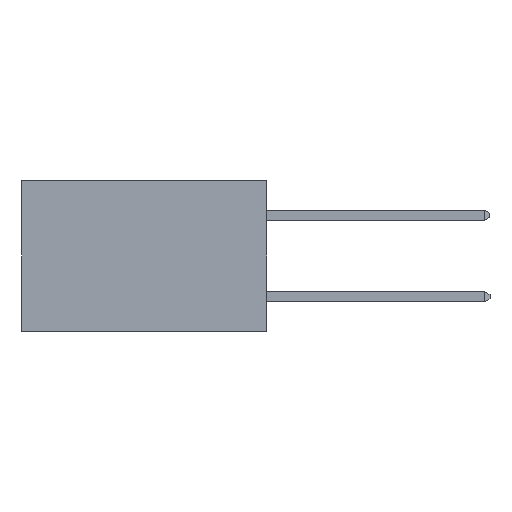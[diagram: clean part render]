
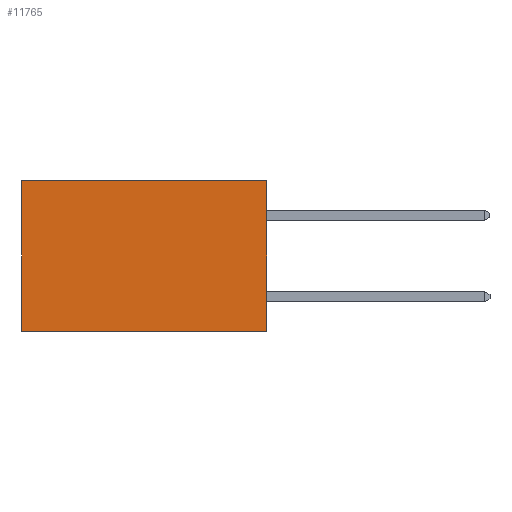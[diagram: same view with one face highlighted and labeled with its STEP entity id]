
A CAD part, left-side view. The second image highlights one B-rep face of the part: STEP entity #11765.
In plain terms, the highlighted planar face has unit normal (-1, 0, 0).
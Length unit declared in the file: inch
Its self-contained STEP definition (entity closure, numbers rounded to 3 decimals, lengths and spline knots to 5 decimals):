
#58 = EDGE_CURVE ( 'NONE', #2391, #2931, #9370, .T. ) ;
#368 = DIRECTION ( 'NONE',  ( 0., 0., -1. ) ) ;
#513 = LINE ( 'NONE', #10757, #8063 ) ;
#1424 = LINE ( 'NONE', #6221, #7368 ) ;
#1634 = EDGE_CURVE ( 'NONE', #2931, #11163, #513, .T. ) ;
#1973 = EDGE_CURVE ( 'NONE', #2391, #8317, #9157, .T. ) ;
#2129 = DIRECTION ( 'NONE',  ( 0., 0., -1. ) ) ;
#2391 = VERTEX_POINT ( 'NONE', #13063 ) ;
#2931 = VERTEX_POINT ( 'NONE', #6387 ) ;
#2952 = CARTESIAN_POINT ( 'NONE',  ( 0.2875, 0., 0. ) ) ;
#3901 = DIRECTION ( 'NONE',  ( 0., 1., 0. ) ) ;
#3923 = VECTOR ( 'NONE', #3943, 39.37008 ) ;
#3943 = DIRECTION ( 'NONE',  ( 0., 0., -1. ) ) ;
#4348 = ORIENTED_EDGE ( 'NONE', *, *, #6949, .T. ) ;
#4667 = DIRECTION ( 'NONE',  ( 1., 0., 0. ) ) ;
#6221 = CARTESIAN_POINT ( 'NONE',  ( 0.2875, 0.6, 0. ) ) ;
#6387 = CARTESIAN_POINT ( 'NONE',  ( 0.2875, 0., -0.37 ) ) ;
#6742 = DIRECTION ( 'NONE',  ( 0., 1., 0. ) ) ;
#6826 = ORIENTED_EDGE ( 'NONE', *, *, #58, .F. ) ;
#6949 = EDGE_CURVE ( 'NONE', #8317, #11163, #1424, .T. ) ;
#7071 = EDGE_LOOP ( 'NONE', ( #4348, #9352, #6826, #9397 ) ) ;
#7368 = VECTOR ( 'NONE', #2129, 39.37008 ) ;
#8063 = VECTOR ( 'NONE', #6742, 39.37008 ) ;
#8317 = VERTEX_POINT ( 'NONE', #9177 ) ;
#9157 = LINE ( 'NONE', #12141, #9624 ) ;
#9177 = CARTESIAN_POINT ( 'NONE',  ( 0.2875, 0.6, 0. ) ) ;
#9352 = ORIENTED_EDGE ( 'NONE', *, *, #1634, .F. ) ;
#9370 = LINE ( 'NONE', #2952, #3923 ) ;
#9397 = ORIENTED_EDGE ( 'NONE', *, *, #1973, .T. ) ;
#9600 = FACE_OUTER_BOUND ( 'NONE', #7071, .T. ) ;
#9624 = VECTOR ( 'NONE', #3901, 39.37008 ) ;
#9629 = AXIS2_PLACEMENT_3D ( 'NONE', #9697, #4667, #368 ) ;
#9697 = CARTESIAN_POINT ( 'NONE',  ( 0.2875, 0., 0. ) ) ;
#10757 = CARTESIAN_POINT ( 'NONE',  ( 0.2875, 0., -0.37 ) ) ;
#10796 = PLANE ( 'NONE',  #9629 ) ;
#11163 = VERTEX_POINT ( 'NONE', #12715 ) ;
#11765 = ADVANCED_FACE ( 'NONE', ( #9600 ), #10796, .F. ) ;
#12141 = CARTESIAN_POINT ( 'NONE',  ( 0.2875, 0., 0. ) ) ;
#12715 = CARTESIAN_POINT ( 'NONE',  ( 0.2875, 0.6, -0.37 ) ) ;
#13063 = CARTESIAN_POINT ( 'NONE',  ( 0.2875, 0., 0. ) ) ;
